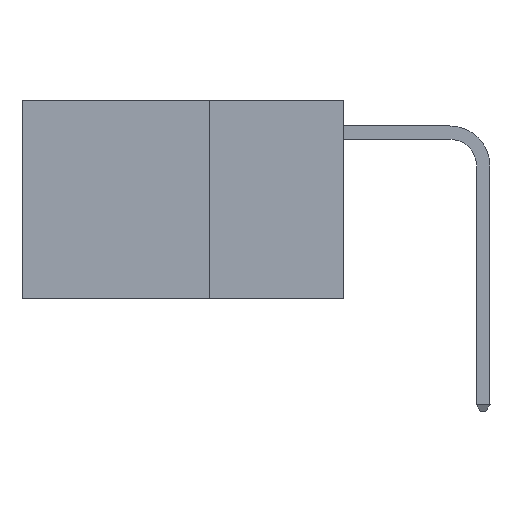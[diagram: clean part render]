
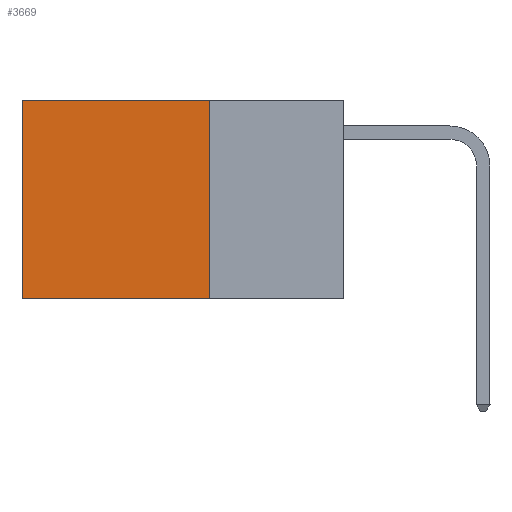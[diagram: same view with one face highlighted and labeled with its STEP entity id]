
A CAD part, left-side view. The second image highlights one B-rep face of the part: STEP entity #3669.
In plain terms, the highlighted planar face has unit normal (-1, 0, 0).
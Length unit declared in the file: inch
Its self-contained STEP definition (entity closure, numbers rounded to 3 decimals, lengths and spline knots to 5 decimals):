
#522 = CARTESIAN_POINT ( 'NONE',  ( 0.2625, 0.6, -0.37 ) ) ;
#903 = CARTESIAN_POINT ( 'NONE',  ( 0.2625, 0.25, 0. ) ) ;
#925 = DIRECTION ( 'NONE',  ( 0., 1., 0. ) ) ;
#1865 = AXIS2_PLACEMENT_3D ( 'NONE', #4277, #4068, #4031 ) ;
#2346 = VERTEX_POINT ( 'NONE', #522 ) ;
#3637 = VERTEX_POINT ( 'NONE', #4764 ) ;
#3669 = ADVANCED_FACE ( 'NONE', ( #7072 ), #4294, .F. ) ;
#4031 = DIRECTION ( 'NONE',  ( 0., 0., -1. ) ) ;
#4068 = DIRECTION ( 'NONE',  ( 1., 0., 0. ) ) ;
#4197 = VERTEX_POINT ( 'NONE', #7082 ) ;
#4237 = EDGE_CURVE ( 'NONE', #3637, #2346, #4896, .T. ) ;
#4277 = CARTESIAN_POINT ( 'NONE',  ( 0.2625, 0.25, 0. ) ) ;
#4294 = PLANE ( 'NONE',  #1865 ) ;
#4305 = VERTEX_POINT ( 'NONE', #6567 ) ;
#4764 = CARTESIAN_POINT ( 'NONE',  ( 0.2625, 0.25, -0.37 ) ) ;
#4882 = VECTOR ( 'NONE', #6843, 39.37008 ) ;
#4896 = LINE ( 'NONE', #6957, #4882 ) ;
#4956 = DIRECTION ( 'NONE',  ( 0., 0., -1. ) ) ;
#5066 = VECTOR ( 'NONE', #925, 39.37008 ) ;
#5188 = LINE ( 'NONE', #903, #5066 ) ;
#5333 = ORIENTED_EDGE ( 'NONE', *, *, #6388, .T. ) ;
#5467 = EDGE_LOOP ( 'NONE', ( #5333, #7291, #8387, #8195 ) ) ;
#5611 = CARTESIAN_POINT ( 'NONE',  ( 0.2625, 0.25, 0. ) ) ;
#6388 = EDGE_CURVE ( 'NONE', #4197, #2346, #7078, .T. ) ;
#6567 = CARTESIAN_POINT ( 'NONE',  ( 0.2625, 0.25, 0. ) ) ;
#6843 = DIRECTION ( 'NONE',  ( 0., 1., 0. ) ) ;
#6957 = CARTESIAN_POINT ( 'NONE',  ( 0.2625, 0.25, -0.37 ) ) ;
#7072 = FACE_OUTER_BOUND ( 'NONE', #5467, .T. ) ;
#7078 = LINE ( 'NONE', #7160, #8623 ) ;
#7082 = CARTESIAN_POINT ( 'NONE',  ( 0.2625, 0.6, 0. ) ) ;
#7160 = CARTESIAN_POINT ( 'NONE',  ( 0.2625, 0.6, 0. ) ) ;
#7192 = DIRECTION ( 'NONE',  ( 0., 0., -1. ) ) ;
#7214 = EDGE_CURVE ( 'NONE', #4305, #4197, #5188, .T. ) ;
#7291 = ORIENTED_EDGE ( 'NONE', *, *, #4237, .F. ) ;
#7417 = VECTOR ( 'NONE', #4956, 39.37008 ) ;
#7425 = LINE ( 'NONE', #5611, #7417 ) ;
#8008 = EDGE_CURVE ( 'NONE', #4305, #3637, #7425, .T. ) ;
#8195 = ORIENTED_EDGE ( 'NONE', *, *, #7214, .T. ) ;
#8387 = ORIENTED_EDGE ( 'NONE', *, *, #8008, .F. ) ;
#8623 = VECTOR ( 'NONE', #7192, 39.37008 ) ;
